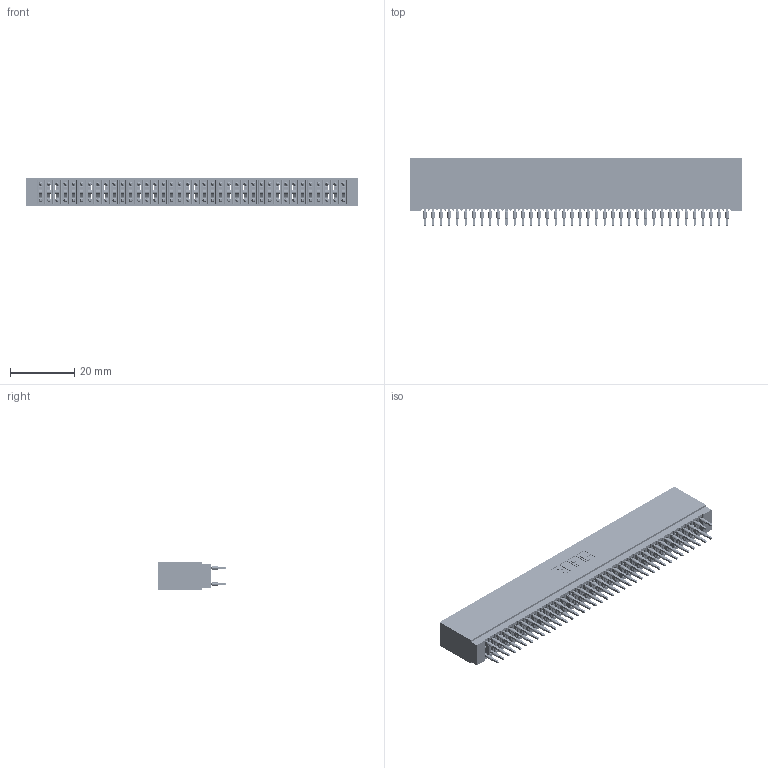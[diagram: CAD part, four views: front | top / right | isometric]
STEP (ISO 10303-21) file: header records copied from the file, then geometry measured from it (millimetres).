
FILE_DESCRIPTION (( 'STEP AP203' ), '1' );
FILE_NAME ('745-076-560-201.STEP', '2026-02-26T20:18:36', ( '' ), ( '' ), 'SwSTEP 2.0', 'SolidWorks 2023', '' );
FILE_SCHEMA (( 'CONFIG_CONTROL_DESIGN' ));
Length unit declared in the file: millimetre
Products named in the file (3): 745-292-001_560; 745 Part_Insulator Option - 01; 745-076-560-201
Assembly tree (77 placements, depth 2):
  745-076-560-201
    745 Part_Insulator Option - 01
    745-292-001_560  x76
Bounding box: 103.12 x 21.22 x 8.89 mm (x, y, z)
Volume: 9592.8 mm3; surface area: 20607 mm2
Topology: 77 solids, 77 shells, 7581 faces, 20740 edges, 13168 vertices
Faces by surface type: plane 3931, cylinder 1674, bspline 1520, torus 456
Entity records: 64843 total; most frequent: CARTESIAN_POINT 11753, ORIENTED_EDGE 11180, DIRECTION 9774, EDGE_CURVE 5590, LINE 5172, VECTOR 5172, VERTEX_POINT 3568, AXIS2_PLACEMENT_3D 2301
